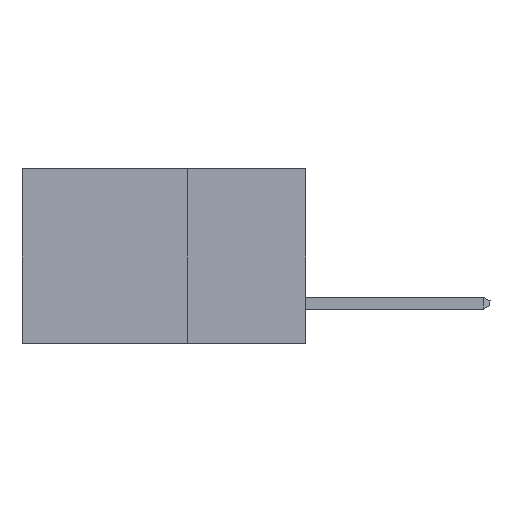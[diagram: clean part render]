
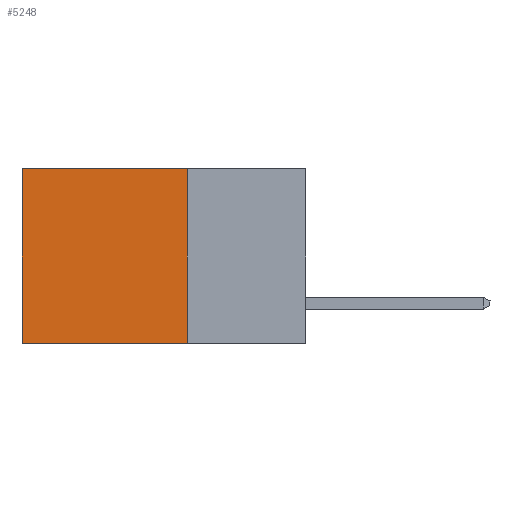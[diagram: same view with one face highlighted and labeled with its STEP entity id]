
A CAD part, left-side view. The second image highlights one B-rep face of the part: STEP entity #5248.
In plain terms, the highlighted planar face has unit normal (-1, 0, 0).
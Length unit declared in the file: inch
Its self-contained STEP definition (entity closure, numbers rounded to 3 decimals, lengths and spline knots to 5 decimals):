
#305 = PLANE ( 'NONE',  #8846 ) ;
#837 = LINE ( 'NONE', #2561, #10476 ) ;
#1912 = CARTESIAN_POINT ( 'NONE',  ( 0.2615, 0.25, -0.37 ) ) ;
#1969 = CARTESIAN_POINT ( 'NONE',  ( 0.2615, 0.6, 0. ) ) ;
#2113 = EDGE_CURVE ( 'NONE', #8564, #5208, #9487, .T. ) ;
#2164 = EDGE_CURVE ( 'NONE', #8564, #5107, #6107, .T. ) ;
#2561 = CARTESIAN_POINT ( 'NONE',  ( 0.2615, 0.6, -0.37 ) ) ;
#3202 = VECTOR ( 'NONE', #9941, 39.37008 ) ;
#3699 = DIRECTION ( 'NONE',  ( 0., 0., -1. ) ) ;
#3903 = CARTESIAN_POINT ( 'NONE',  ( 0.2615, 0.25, -0.37 ) ) ;
#4441 = DIRECTION ( 'NONE',  ( 0., 0., -1. ) ) ;
#5107 = VERTEX_POINT ( 'NONE', #8475 ) ;
#5208 = VERTEX_POINT ( 'NONE', #1969 ) ;
#5248 = ADVANCED_FACE ( 'NONE', ( #9526 ), #305, .F. ) ;
#6107 = LINE ( 'NONE', #8649, #9850 ) ;
#6310 = VERTEX_POINT ( 'NONE', #7813 ) ;
#7102 = ORIENTED_EDGE ( 'NONE', *, *, #7215, .T. ) ;
#7215 = EDGE_CURVE ( 'NONE', #5208, #6310, #837, .T. ) ;
#7385 = ORIENTED_EDGE ( 'NONE', *, *, #2113, .T. ) ;
#7519 = EDGE_CURVE ( 'NONE', #5107, #6310, #9830, .T. ) ;
#7813 = CARTESIAN_POINT ( 'NONE',  ( 0.2615, 0.6, -0.37 ) ) ;
#7871 = ORIENTED_EDGE ( 'NONE', *, *, #7519, .F. ) ;
#7877 = CARTESIAN_POINT ( 'NONE',  ( 0.2615, 0.25, 0. ) ) ;
#8475 = CARTESIAN_POINT ( 'NONE',  ( 0.2615, 0.25, -0.37 ) ) ;
#8522 = ORIENTED_EDGE ( 'NONE', *, *, #2164, .F. ) ;
#8564 = VERTEX_POINT ( 'NONE', #9457 ) ;
#8625 = VECTOR ( 'NONE', #8813, 39.37008 ) ;
#8649 = CARTESIAN_POINT ( 'NONE',  ( 0.2615, 0.25, -0.37 ) ) ;
#8813 = DIRECTION ( 'NONE',  ( 0., 1., 0. ) ) ;
#8846 = AXIS2_PLACEMENT_3D ( 'NONE', #1912, #9688, #3699 ) ;
#8947 = EDGE_LOOP ( 'NONE', ( #7102, #7871, #8522, #7385 ) ) ;
#9454 = DIRECTION ( 'NONE',  ( 0., 0., -1. ) ) ;
#9457 = CARTESIAN_POINT ( 'NONE',  ( 0.2615, 0.25, 0. ) ) ;
#9487 = LINE ( 'NONE', #7877, #8625 ) ;
#9526 = FACE_OUTER_BOUND ( 'NONE', #8947, .T. ) ;
#9688 = DIRECTION ( 'NONE',  ( 1., 0., 0. ) ) ;
#9830 = LINE ( 'NONE', #3903, #3202 ) ;
#9850 = VECTOR ( 'NONE', #4441, 39.37008 ) ;
#9941 = DIRECTION ( 'NONE',  ( 0., 1., 0. ) ) ;
#10476 = VECTOR ( 'NONE', #9454, 39.37008 ) ;
